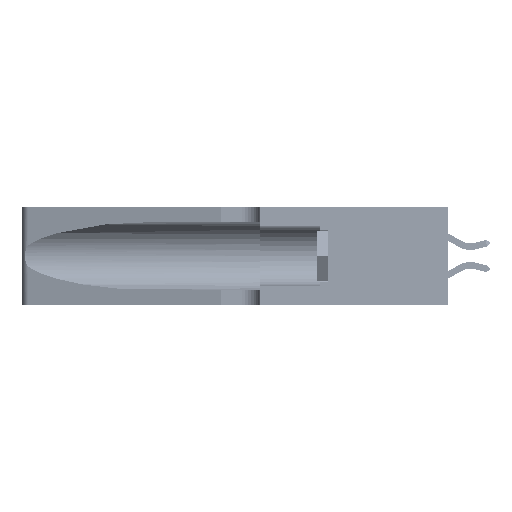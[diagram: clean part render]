
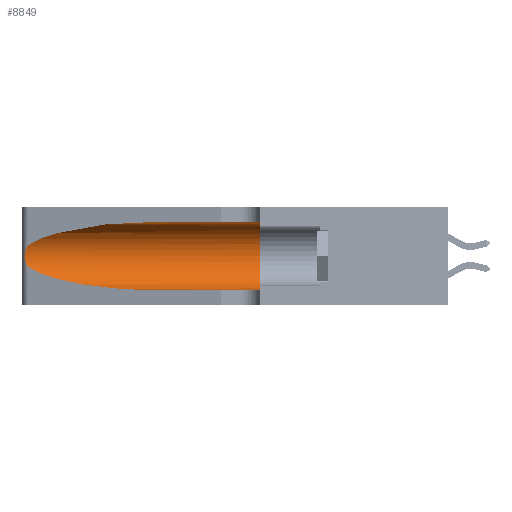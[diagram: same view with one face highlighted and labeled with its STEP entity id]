
A CAD part, left-side view. The second image highlights one B-rep face of the part: STEP entity #8849.
In plain terms, the highlighted cylindrical face has radius 3.308 mm (diameter 6.617 mm), a partial arc.
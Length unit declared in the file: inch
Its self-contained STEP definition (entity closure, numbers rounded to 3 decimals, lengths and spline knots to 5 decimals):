
#682 = CARTESIAN_POINT ( 'NONE',  ( 0.26017, 1.23833, 0.17102 ) ) ;
#1587 = ORIENTED_EDGE ( 'NONE', *, *, #23776, .F. ) ;
#1645 = ORIENTED_EDGE ( 'NONE', *, *, #4599, .F. ) ;
#2826 = ORIENTED_EDGE ( 'NONE', *, *, #36850, .T. ) ;
#3878 = DIRECTION ( 'NONE',  ( 0., -1., 0. ) ) ;
#3979 =( BOUNDED_CURVE ( )  B_SPLINE_CURVE ( 3, ( #11835, #33931, #37598, #15569 ),
 .UNSPECIFIED., .F., .T. ) 
 B_SPLINE_CURVE_WITH_KNOTS ( ( 4, 4 ),
 ( 1.5708, 2.84003 ),
 .UNSPECIFIED. ) 
 CURVE ( )  GEOMETRIC_REPRESENTATION_ITEM ( )  RATIONAL_B_SPLINE_CURVE ( ( 1., 0.87, 0.87, 1. ) ) 
 REPRESENTATION_ITEM ( '' )  );
#4254 = EDGE_CURVE ( 'NONE', #38704, #24143, #3979, .T. ) ;
#4290 = CARTESIAN_POINT ( 'NONE',  ( 0.25487, 1.22718, 0.22369 ) ) ;
#4459 = CARTESIAN_POINT ( 'NONE',  ( 0.25789, 1.23486, 0.15765 ) ) ;
#4599 = EDGE_CURVE ( 'NONE', #38704, #18546, #39884, .T. ) ;
#5775 = CARTESIAN_POINT ( 'NONE',  ( 0.25487, 1.22718, 0.14631 ) ) ;
#6540 = CARTESIAN_POINT ( 'NONE',  ( 0.1305, 1.61858, 0.31525 ) ) ;
#7161 = VERTEX_POINT ( 'NONE', #29008 ) ;
#7634 = LINE ( 'NONE', #37047, #16439 ) ;
#8053 = CARTESIAN_POINT ( 'NONE',  ( 0.25555, 1.22994, 0.2215 ) ) ;
#8218 = CARTESIAN_POINT ( 'NONE',  ( 0.25555, 1.22993, 0.14849 ) ) ;
#8849 = ADVANCED_FACE ( 'NONE', ( #15093 ), #13951, .F. ) ;
#11835 = CARTESIAN_POINT ( 'NONE',  ( 0.1305, 0.72297, 0.31525 ) ) ;
#12085 = AXIS2_PLACEMENT_3D ( 'NONE', #34573, #12484, #38251 ) ;
#12484 = DIRECTION ( 'NONE',  ( 0., 1., 0. ) ) ;
#12494 = VERTEX_POINT ( 'NONE', #23096 ) ;
#13339 = CARTESIAN_POINT ( 'NONE',  ( 0.18966, 0.96281, 0.05475 ) ) ;
#13951 = CYLINDRICAL_SURFACE ( 'NONE', #16370, 0.13025 ) ;
#14200 =( BOUNDED_CURVE ( )  B_SPLINE_CURVE ( 3, ( #5775, #28083, #13339, #39077 ),
 .UNSPECIFIED., .F., .F. ) 
 B_SPLINE_CURVE_WITH_KNOTS ( ( 4, 4 ),
 ( 3.44316, 4.71239 ),
 .UNSPECIFIED. ) 
 CURVE ( )  GEOMETRIC_REPRESENTATION_ITEM ( )  RATIONAL_B_SPLINE_CURVE ( ( 1., 0.87, 0.87, 1. ) ) 
 REPRESENTATION_ITEM ( '' )  );
#15093 = FACE_OUTER_BOUND ( 'NONE', #22166, .T. ) ;
#15569 = CARTESIAN_POINT ( 'NONE',  ( 0.25487, 1.22718, 0.22369 ) ) ;
#15590 = CARTESIAN_POINT ( 'NONE',  ( 0.25787, 1.23484, 0.2124 ) ) ;
#16224 = CARTESIAN_POINT ( 'NONE',  ( 0.1305, 1.61858, 0.185 ) ) ;
#16370 = AXIS2_PLACEMENT_3D ( 'NONE', #16224, #45578, #34560 ) ;
#16439 = VECTOR ( 'NONE', #3878, 39.37008 ) ;
#17462 = ORIENTED_EDGE ( 'NONE', *, *, #35894, .T. ) ;
#18546 = VERTEX_POINT ( 'NONE', #25867 ) ;
#19307 = CARTESIAN_POINT ( 'NONE',  ( 0.26018, 1.23835, 0.19895 ) ) ;
#22166 = EDGE_LOOP ( 'NONE', ( #29405, #29591, #17462, #2826, #1587, #1645 ) ) ;
#23048 = CARTESIAN_POINT ( 'NONE',  ( 0.26075, 1.23896, 0.178 ) ) ;
#23096 = CARTESIAN_POINT ( 'NONE',  ( 0.25487, 1.22718, 0.14631 ) ) ;
#23776 = EDGE_CURVE ( 'NONE', #18546, #7161, #39907, .T. ) ;
#24143 = VERTEX_POINT ( 'NONE', #29163 ) ;
#25867 = CARTESIAN_POINT ( 'NONE',  ( 0.1305, 0.35, 0.31525 ) ) ;
#26753 = CARTESIAN_POINT ( 'NONE',  ( 0.25856, 1.23593, 0.16098 ) ) ;
#28083 = CARTESIAN_POINT ( 'NONE',  ( 0.2373, 1.15595, 0.08982 ) ) ;
#29008 = CARTESIAN_POINT ( 'NONE',  ( 0.1305, 0.35, 0.05475 ) ) ;
#29163 = CARTESIAN_POINT ( 'NONE',  ( 0.25487, 1.22718, 0.22369 ) ) ;
#29227 = CARTESIAN_POINT ( 'NONE',  ( 0.1305, 0.72297, 0.31525 ) ) ;
#29405 = ORIENTED_EDGE ( 'NONE', *, *, #4254, .T. ) ;
#29591 = ORIENTED_EDGE ( 'NONE', *, *, #33508, .T. ) ;
#30484 = CARTESIAN_POINT ( 'NONE',  ( 0.25639, 1.23186, 0.15144 ) ) ;
#31400 = B_SPLINE_CURVE_WITH_KNOTS ( 'NONE', 3,
 ( #4290, #8053, #37615, #15590, #41280, #19307, #44951, #23048, #682, #26753, #4459, #30484, #8218, #34110 ),
 .UNSPECIFIED., .F., .F.,
 ( 4, 2, 2, 2, 2, 2, 4 ),
 ( 0., 0.00027, 0.00053, 0.00107, 0.0016, 0.00187, 0.00214 ),
 .UNSPECIFIED. ) ;
#32513 = DIRECTION ( 'NONE',  ( 0., -1., 0. ) ) ;
#33508 = EDGE_CURVE ( 'NONE', #24143, #12494, #31400, .T. ) ;
#33931 = CARTESIAN_POINT ( 'NONE',  ( 0.18966, 0.96281, 0.31525 ) ) ;
#34110 = CARTESIAN_POINT ( 'NONE',  ( 0.25487, 1.22718, 0.14631 ) ) ;
#34560 = DIRECTION ( 'NONE',  ( 0., 0., -1. ) ) ;
#34573 = CARTESIAN_POINT ( 'NONE',  ( 0.1305, 0.35, 0.185 ) ) ;
#35894 = EDGE_CURVE ( 'NONE', #12494, #38591, #14200, .T. ) ;
#36850 = EDGE_CURVE ( 'NONE', #38591, #7161, #7634, .T. ) ;
#37047 = CARTESIAN_POINT ( 'NONE',  ( 0.1305, 1.61858, 0.05475 ) ) ;
#37598 = CARTESIAN_POINT ( 'NONE',  ( 0.2373, 1.15595, 0.28018 ) ) ;
#37615 = CARTESIAN_POINT ( 'NONE',  ( 0.25639, 1.23184, 0.21858 ) ) ;
#38251 = DIRECTION ( 'NONE',  ( 0., 0., 1. ) ) ;
#38591 = VERTEX_POINT ( 'NONE', #43235 ) ;
#38704 = VERTEX_POINT ( 'NONE', #29227 ) ;
#38740 = VECTOR ( 'NONE', #32513, 39.37008 ) ;
#39077 = CARTESIAN_POINT ( 'NONE',  ( 0.1305, 0.72297, 0.05475 ) ) ;
#39884 = LINE ( 'NONE', #6540, #38740 ) ;
#39907 = CIRCLE ( 'NONE', #12085, 0.13025 ) ;
#41280 = CARTESIAN_POINT ( 'NONE',  ( 0.25854, 1.2359, 0.20912 ) ) ;
#43235 = CARTESIAN_POINT ( 'NONE',  ( 0.1305, 0.72297, 0.05475 ) ) ;
#44951 = CARTESIAN_POINT ( 'NONE',  ( 0.26075, 1.23896, 0.19203 ) ) ;
#45578 = DIRECTION ( 'NONE',  ( 0., -1., 0. ) ) ;
